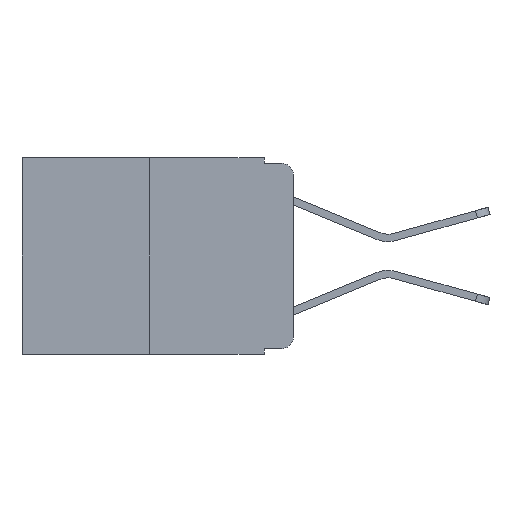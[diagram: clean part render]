
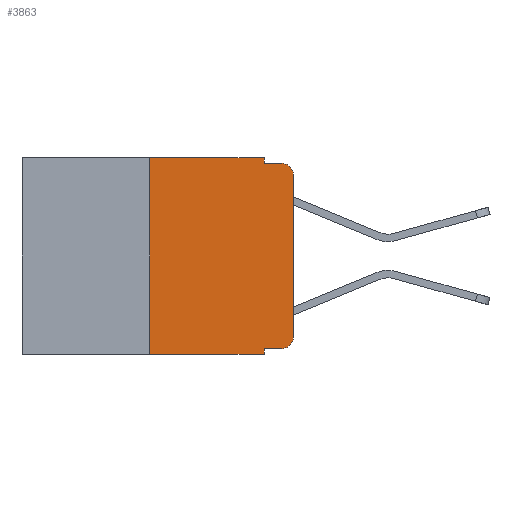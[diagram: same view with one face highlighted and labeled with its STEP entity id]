
A CAD part, left-side view. The second image highlights one B-rep face of the part: STEP entity #3863.
In plain terms, the highlighted planar face has unit normal (-1, 0, 0).
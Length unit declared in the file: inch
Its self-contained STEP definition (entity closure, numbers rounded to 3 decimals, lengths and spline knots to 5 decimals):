
#229 = VECTOR ( 'NONE', #15286, 39.37008 ) ;
#636 = AXIS2_PLACEMENT_3D ( 'NONE', #14781, #6512, #16131 ) ;
#680 = LINE ( 'NONE', #12641, #229 ) ;
#813 = LINE ( 'NONE', #3220, #3759 ) ;
#825 = LINE ( 'NONE', #10272, #7925 ) ;
#835 = DIRECTION ( 'NONE',  ( 0., 0., 1. ) ) ;
#880 = EDGE_CURVE ( 'NONE', #9997, #8871, #17057, .T. ) ;
#891 = FACE_OUTER_BOUND ( 'NONE', #3976, .T. ) ;
#1296 = ORIENTED_EDGE ( 'NONE', *, *, #17213, .T. ) ;
#1408 = EDGE_CURVE ( 'NONE', #7319, #15655, #4335, .T. ) ;
#1595 = VERTEX_POINT ( 'NONE', #16599 ) ;
#2024 = CARTESIAN_POINT ( 'NONE',  ( 0., 0., -0.03 ) ) ;
#2502 = AXIS2_PLACEMENT_3D ( 'NONE', #10384, #12989, #13012 ) ;
#2755 = VECTOR ( 'NONE', #6423, 39.37008 ) ;
#3084 = ORIENTED_EDGE ( 'NONE', *, *, #880, .T. ) ;
#3220 = CARTESIAN_POINT ( 'NONE',  ( 0., 0.473, -0.343 ) ) ;
#3325 = ORIENTED_EDGE ( 'NONE', *, *, #14046, .T. ) ;
#3604 = CARTESIAN_POINT ( 'NONE',  ( 0., 0.051, -0.01 ) ) ;
#3759 = VECTOR ( 'NONE', #12973, 39.37008 ) ;
#3782 = ORIENTED_EDGE ( 'NONE', *, *, #9527, .F. ) ;
#3863 = ADVANCED_FACE ( 'NONE', ( #891 ), #9104, .F. ) ;
#3976 = EDGE_LOOP ( 'NONE', ( #3084, #7717, #11821, #8574, #13126, #10322, #3325, #3782, #4215, #1296 ) ) ;
#4215 = ORIENTED_EDGE ( 'NONE', *, *, #13561, .T. ) ;
#4335 = LINE ( 'NONE', #17330, #7621 ) ;
#4748 = EDGE_CURVE ( 'NONE', #8871, #1595, #16909, .T. ) ;
#5062 = VERTEX_POINT ( 'NONE', #12815 ) ;
#5541 = EDGE_CURVE ( 'NONE', #15655, #5062, #6379, .T. ) ;
#5640 = CARTESIAN_POINT ( 'NONE',  ( 0., 0.051, -0.343 ) ) ;
#6379 = LINE ( 'NONE', #10828, #7263 ) ;
#6423 = DIRECTION ( 'NONE',  ( 0., 0., -1. ) ) ;
#6512 = DIRECTION ( 'NONE',  ( -1., 0., 0. ) ) ;
#6964 = VERTEX_POINT ( 'NONE', #14342 ) ;
#7263 = VECTOR ( 'NONE', #10711, 39.37008 ) ;
#7319 = VERTEX_POINT ( 'NONE', #11898 ) ;
#7367 = AXIS2_PLACEMENT_3D ( 'NONE', #8905, #9060, #8968 ) ;
#7621 = VECTOR ( 'NONE', #8419, 39.37008 ) ;
#7717 = ORIENTED_EDGE ( 'NONE', *, *, #4748, .T. ) ;
#7925 = VECTOR ( 'NONE', #14419, 39.37008 ) ;
#8419 = DIRECTION ( 'NONE',  ( 0., -1., 0. ) ) ;
#8574 = ORIENTED_EDGE ( 'NONE', *, *, #5541, .F. ) ;
#8871 = VERTEX_POINT ( 'NONE', #2024 ) ;
#8879 = CIRCLE ( 'NONE', #636, 0.02 ) ;
#8905 = CARTESIAN_POINT ( 'NONE',  ( 0., 0.473, 0. ) ) ;
#8968 = DIRECTION ( 'NONE',  ( 0., 0., -1. ) ) ;
#9060 = DIRECTION ( 'NONE',  ( 1., 0., 0. ) ) ;
#9104 = PLANE ( 'NONE',  #7367 ) ;
#9238 = CARTESIAN_POINT ( 'NONE',  ( 0., 0.051, 0. ) ) ;
#9402 = VECTOR ( 'NONE', #835, 39.37008 ) ;
#9527 = EDGE_CURVE ( 'NONE', #9575, #15690, #17013, .T. ) ;
#9575 = VERTEX_POINT ( 'NONE', #17434 ) ;
#9997 = VERTEX_POINT ( 'NONE', #11625 ) ;
#10272 = CARTESIAN_POINT ( 'NONE',  ( 0., 0.051, -0.333 ) ) ;
#10322 = ORIENTED_EDGE ( 'NONE', *, *, #17439, .F. ) ;
#10384 = CARTESIAN_POINT ( 'NONE',  ( 0., 0.02, -0.03 ) ) ;
#10675 = CARTESIAN_POINT ( 'NONE',  ( 0., 0., 0. ) ) ;
#10711 = DIRECTION ( 'NONE',  ( 0., 0., -1. ) ) ;
#10828 = CARTESIAN_POINT ( 'NONE',  ( 0., 0.051, 0. ) ) ;
#11625 = CARTESIAN_POINT ( 'NONE',  ( 0., 0., -0.313 ) ) ;
#11821 = ORIENTED_EDGE ( 'NONE', *, *, #12418, .F. ) ;
#11898 = CARTESIAN_POINT ( 'NONE',  ( 0., 0.25, 0. ) ) ;
#12418 = EDGE_CURVE ( 'NONE', #5062, #1595, #16701, .T. ) ;
#12641 = CARTESIAN_POINT ( 'NONE',  ( 0., 0.25, 0. ) ) ;
#12815 = CARTESIAN_POINT ( 'NONE',  ( 0., 0.051, -0.01 ) ) ;
#12973 = DIRECTION ( 'NONE',  ( 0., -1., 0. ) ) ;
#12989 = DIRECTION ( 'NONE',  ( -1., 0., 0. ) ) ;
#13012 = DIRECTION ( 'NONE',  ( 0., 0., -1. ) ) ;
#13126 = ORIENTED_EDGE ( 'NONE', *, *, #1408, .F. ) ;
#13145 = VERTEX_POINT ( 'NONE', #16121 ) ;
#13149 = VECTOR ( 'NONE', #14687, 39.37008 ) ;
#13561 = EDGE_CURVE ( 'NONE', #9575, #6964, #825, .T. ) ;
#14046 = EDGE_CURVE ( 'NONE', #13145, #15690, #813, .T. ) ;
#14342 = CARTESIAN_POINT ( 'NONE',  ( 0., 0.02, -0.333 ) ) ;
#14419 = DIRECTION ( 'NONE',  ( 0., -1., 0. ) ) ;
#14687 = DIRECTION ( 'NONE',  ( 0., -1., 0. ) ) ;
#14781 = CARTESIAN_POINT ( 'NONE',  ( 0., 0.02, -0.313 ) ) ;
#15286 = DIRECTION ( 'NONE',  ( 0., 0., 1. ) ) ;
#15655 = VERTEX_POINT ( 'NONE', #17730 ) ;
#15690 = VERTEX_POINT ( 'NONE', #5640 ) ;
#16121 = CARTESIAN_POINT ( 'NONE',  ( 0., 0.25, -0.343 ) ) ;
#16131 = DIRECTION ( 'NONE',  ( 0., 0., -1. ) ) ;
#16599 = CARTESIAN_POINT ( 'NONE',  ( 0., 0.02, -0.01 ) ) ;
#16701 = LINE ( 'NONE', #3604, #13149 ) ;
#16909 = CIRCLE ( 'NONE', #2502, 0.02 ) ;
#17013 = LINE ( 'NONE', #9238, #2755 ) ;
#17057 = LINE ( 'NONE', #10675, #9402 ) ;
#17213 = EDGE_CURVE ( 'NONE', #6964, #9997, #8879, .T. ) ;
#17330 = CARTESIAN_POINT ( 'NONE',  ( 0., 0.473, 0. ) ) ;
#17434 = CARTESIAN_POINT ( 'NONE',  ( 0., 0.051, -0.333 ) ) ;
#17439 = EDGE_CURVE ( 'NONE', #13145, #7319, #680, .T. ) ;
#17730 = CARTESIAN_POINT ( 'NONE',  ( 0., 0.051, 0. ) ) ;
